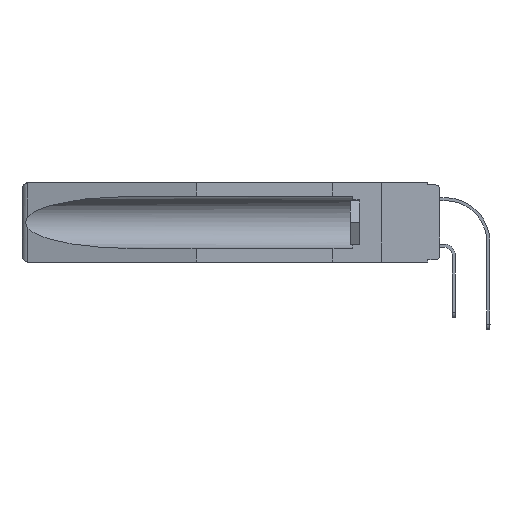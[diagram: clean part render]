
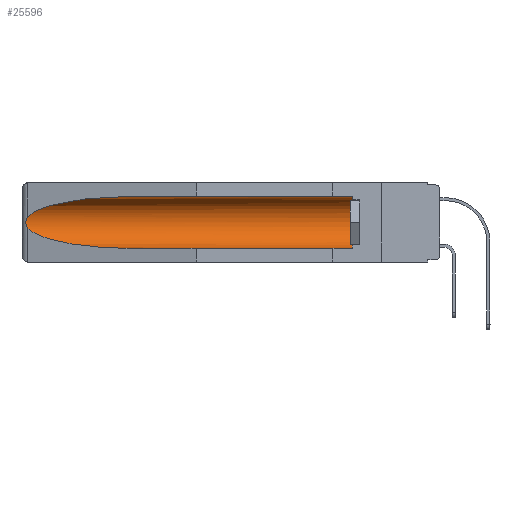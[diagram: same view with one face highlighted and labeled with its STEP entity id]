
A CAD part, left-side view. The second image highlights one B-rep face of the part: STEP entity #25596.
In plain terms, the highlighted cylindrical face has radius 2.857 mm (diameter 5.715 mm), a partial arc.
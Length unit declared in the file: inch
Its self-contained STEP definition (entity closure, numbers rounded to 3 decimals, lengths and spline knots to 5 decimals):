
#568 = EDGE_CURVE ( 'NONE', #10303, #6135, #16099, .T. ) ;
#1346 = B_SPLINE_CURVE_WITH_KNOTS ( 'NONE', 3,
 ( #12599, #28569, #7924, #27354, #22212, #10935, #18158, #20405, #1892, #2191 ),
 .UNSPECIFIED., .F., .F.,
 ( 4, 2, 2, 2, 4 ),
 ( 0., 0.00029, 0.00058, 0.00087, 0.00117 ),
 .UNSPECIFIED. ) ;
#1892 = CARTESIAN_POINT ( 'NONE',  ( 0.26597, 1.5296, -0.19026 ) ) ;
#2191 = CARTESIAN_POINT ( 'NONE',  ( 0.26537, 1.52718, -0.19328 ) ) ;
#2511 = AXIS2_PLACEMENT_3D ( 'NONE', #5171, #14348, #19162 ) ;
#2527 = CARTESIAN_POINT ( 'NONE',  ( 0.155, 1.07973, -0.059 ) ) ;
#2685 = CARTESIAN_POINT ( 'NONE',  ( 0.26537, 1.52718, -0.14972 ) ) ;
#2767 = CARTESIAN_POINT ( 'NONE',  ( 0.155, 1.07973, -0.284 ) ) ;
#4620 = EDGE_CURVE ( 'NONE', #6135, #29105, #1346, .T. ) ;
#5171 = CARTESIAN_POINT ( 'NONE',  ( 0.155, 0.126, -0.1715 ) ) ;
#5495 = CARTESIAN_POINT ( 'NONE',  ( 0.155, 1.07973, -0.284 ) ) ;
#6135 = VERTEX_POINT ( 'NONE', #21013 ) ;
#6692 =( BOUNDED_CURVE ( )  B_SPLINE_CURVE ( 3, ( #24331, #14973, #12442, #5495 ),
 .UNSPECIFIED., .F., .T. ) 
 B_SPLINE_CURVE_WITH_KNOTS ( ( 4, 4 ),
 ( 0.1948, 1.5708 ),
 .UNSPECIFIED. ) 
 CURVE ( )  GEOMETRIC_REPRESENTATION_ITEM ( )  RATIONAL_B_SPLINE_CURVE ( ( 1., 0.848, 0.848, 1. ) ) 
 REPRESENTATION_ITEM ( '' )  );
#7924 = CARTESIAN_POINT ( 'NONE',  ( 0.26654, 1.53092, -0.15636 ) ) ;
#9914 = VECTOR ( 'NONE', #12643, 39.37008 ) ;
#10046 = DIRECTION ( 'NONE',  ( 0., 0., 1. ) ) ;
#10215 = LINE ( 'NONE', #29072, #9914 ) ;
#10303 = VERTEX_POINT ( 'NONE', #19234 ) ;
#10935 = CARTESIAN_POINT ( 'NONE',  ( 0.2675, 1.53308, -0.17534 ) ) ;
#11728 = CARTESIAN_POINT ( 'NONE',  ( 0.25451, 1.48313, -0.09465 ) ) ;
#12442 = CARTESIAN_POINT ( 'NONE',  ( 0.21114, 1.30732, -0.284 ) ) ;
#12471 = DIRECTION ( 'NONE',  ( 0., 1., 0. ) ) ;
#12599 = CARTESIAN_POINT ( 'NONE',  ( 0.26537, 1.52718, -0.14972 ) ) ;
#12643 = DIRECTION ( 'NONE',  ( 0., 1., 0. ) ) ;
#13061 = FACE_OUTER_BOUND ( 'NONE', #28616, .T. ) ;
#14348 = DIRECTION ( 'NONE',  ( 0., -1., 0. ) ) ;
#14351 = LINE ( 'NONE', #25946, #16539 ) ;
#14973 = CARTESIAN_POINT ( 'NONE',  ( 0.25451, 1.48313, -0.24835 ) ) ;
#14994 = CIRCLE ( 'NONE', #2511, 0.1125 ) ;
#15000 = CYLINDRICAL_SURFACE ( 'NONE', #20034, 0.1125 ) ;
#15683 = VERTEX_POINT ( 'NONE', #22800 ) ;
#15784 = EDGE_CURVE ( 'NONE', #19886, #15683, #14994, .T. ) ;
#16099 =( BOUNDED_CURVE ( )  B_SPLINE_CURVE ( 3, ( #2527, #21052, #11728, #2685 ),
 .UNSPECIFIED., .F., .T. ) 
 B_SPLINE_CURVE_WITH_KNOTS ( ( 4, 4 ),
 ( 4.71239, 6.08839 ),
 .UNSPECIFIED. ) 
 CURVE ( )  GEOMETRIC_REPRESENTATION_ITEM ( )  RATIONAL_B_SPLINE_CURVE ( ( 1., 0.848, 0.848, 1. ) ) 
 REPRESENTATION_ITEM ( '' )  );
#16539 = VECTOR ( 'NONE', #17061, 39.37008 ) ;
#17010 = EDGE_CURVE ( 'NONE', #15683, #10303, #14351, .T. ) ;
#17061 = DIRECTION ( 'NONE',  ( 0., 1., 0. ) ) ;
#18158 = CARTESIAN_POINT ( 'NONE',  ( 0.2673, 1.53269, -0.17917 ) ) ;
#19117 = ORIENTED_EDGE ( 'NONE', *, *, #568, .T. ) ;
#19162 = DIRECTION ( 'NONE',  ( 0., 0., 1. ) ) ;
#19234 = CARTESIAN_POINT ( 'NONE',  ( 0.155, 1.07973, -0.059 ) ) ;
#19597 = ORIENTED_EDGE ( 'NONE', *, *, #27394, .T. ) ;
#19886 = VERTEX_POINT ( 'NONE', #26293 ) ;
#20034 = AXIS2_PLACEMENT_3D ( 'NONE', #28437, #12471, #10046 ) ;
#20405 = CARTESIAN_POINT ( 'NONE',  ( 0.26655, 1.53094, -0.18657 ) ) ;
#21013 = CARTESIAN_POINT ( 'NONE',  ( 0.26537, 1.52718, -0.14972 ) ) ;
#21052 = CARTESIAN_POINT ( 'NONE',  ( 0.21114, 1.30732, -0.059 ) ) ;
#22212 = CARTESIAN_POINT ( 'NONE',  ( 0.2675, 1.53308, -0.16763 ) ) ;
#22800 = CARTESIAN_POINT ( 'NONE',  ( 0.155, 0.126, -0.059 ) ) ;
#23265 = CARTESIAN_POINT ( 'NONE',  ( 0.26537, 1.52718, -0.19328 ) ) ;
#24331 = CARTESIAN_POINT ( 'NONE',  ( 0.26537, 1.52718, -0.19328 ) ) ;
#24385 = ORIENTED_EDGE ( 'NONE', *, *, #17010, .T. ) ;
#25173 = EDGE_CURVE ( 'NONE', #19886, #26309, #10215, .T. ) ;
#25596 = ADVANCED_FACE ( 'NONE', ( #13061 ), #15000, .F. ) ;
#25929 = ORIENTED_EDGE ( 'NONE', *, *, #15784, .T. ) ;
#25946 = CARTESIAN_POINT ( 'NONE',  ( 0.155, -0.30754, -0.059 ) ) ;
#26293 = CARTESIAN_POINT ( 'NONE',  ( 0.155, 0.126, -0.284 ) ) ;
#26309 = VERTEX_POINT ( 'NONE', #2767 ) ;
#26384 = ORIENTED_EDGE ( 'NONE', *, *, #25173, .F. ) ;
#27354 = CARTESIAN_POINT ( 'NONE',  ( 0.2673, 1.5327, -0.16383 ) ) ;
#27394 = EDGE_CURVE ( 'NONE', #29105, #26309, #6692, .T. ) ;
#28437 = CARTESIAN_POINT ( 'NONE',  ( 0.155, -0.30754, -0.1715 ) ) ;
#28569 = CARTESIAN_POINT ( 'NONE',  ( 0.26597, 1.52961, -0.15275 ) ) ;
#28616 = EDGE_LOOP ( 'NONE', ( #19117, #29114, #19597, #26384, #25929, #24385 ) ) ;
#29072 = CARTESIAN_POINT ( 'NONE',  ( 0.155, -0.30754, -0.284 ) ) ;
#29105 = VERTEX_POINT ( 'NONE', #23265 ) ;
#29114 = ORIENTED_EDGE ( 'NONE', *, *, #4620, .T. ) ;
